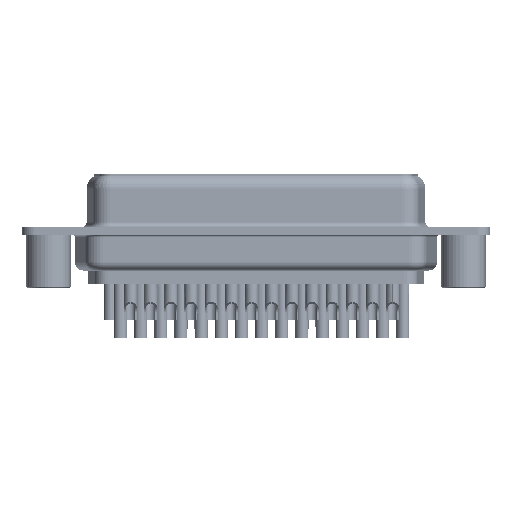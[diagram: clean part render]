
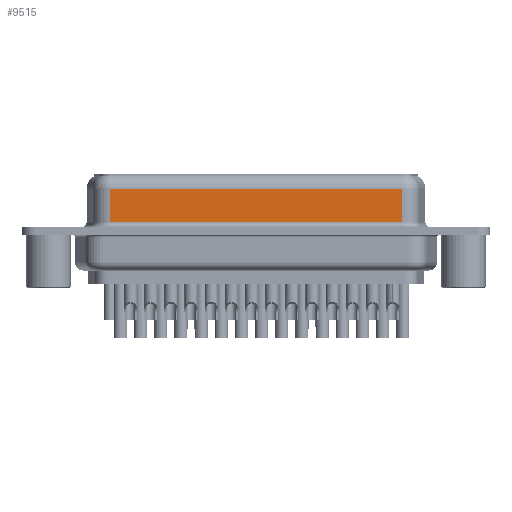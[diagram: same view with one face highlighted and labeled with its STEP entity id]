
A CAD part, front view. The second image highlights one B-rep face of the part: STEP entity #9515.
In plain terms, the highlighted planar face has unit normal (0, -1, 0).
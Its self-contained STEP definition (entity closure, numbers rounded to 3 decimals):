
#59 = CARTESIAN_POINT ( 'NONE',  ( 7.008, -3.95, 0.95 ) ) ;
#691 = DIRECTION ( 'NONE',  ( 0., 0., 1. ) ) ;
#1302 = EDGE_LOOP ( 'NONE', ( #9864, #17698, #5808, #7569 ) ) ;
#1887 = VECTOR ( 'NONE', #4143, 1000. ) ;
#4143 = DIRECTION ( 'NONE',  ( 0., 0., -1. ) ) ;
#5808 = ORIENTED_EDGE ( 'NONE', *, *, #12769, .T. ) ;
#6657 = EDGE_CURVE ( 'NONE', #9003, #11045, #10834, .T. ) ;
#7569 = ORIENTED_EDGE ( 'NONE', *, *, #13275, .T. ) ;
#9003 = VERTEX_POINT ( 'NONE', #17481 ) ;
#9515 = ADVANCED_FACE ( 'NONE', ( #14064 ), #31377, .F. ) ;
#9864 = ORIENTED_EDGE ( 'NONE', *, *, #21808, .F. ) ;
#10677 = VECTOR ( 'NONE', #25814, 1000. ) ;
#10834 = LINE ( 'NONE', #31301, #27037 ) ;
#11045 = VERTEX_POINT ( 'NONE', #33156 ) ;
#11209 = DIRECTION ( 'NONE',  ( -1., 0., 0. ) ) ;
#12769 = EDGE_CURVE ( 'NONE', #11045, #16908, #17257, .T. ) ;
#13275 = EDGE_CURVE ( 'NONE', #16908, #16281, #23882, .T. ) ;
#14064 = FACE_OUTER_BOUND ( 'NONE', #1302, .T. ) ;
#16281 = VERTEX_POINT ( 'NONE', #36037 ) ;
#16908 = VERTEX_POINT ( 'NONE', #59 ) ;
#17257 = LINE ( 'NONE', #30852, #10677 ) ;
#17427 = DIRECTION ( 'NONE',  ( 0., 1., 0. ) ) ;
#17481 = CARTESIAN_POINT ( 'NONE',  ( 40.032, -3.95, 4.7 ) ) ;
#17698 = ORIENTED_EDGE ( 'NONE', *, *, #6657, .T. ) ;
#18462 = LINE ( 'NONE', #24735, #1887 ) ;
#21808 = EDGE_CURVE ( 'NONE', #9003, #16281, #18462, .T. ) ;
#23150 = CARTESIAN_POINT ( 'NONE',  ( 40.032, -3.95, 0.95 ) ) ;
#23882 = LINE ( 'NONE', #23150, #28459 ) ;
#24735 = CARTESIAN_POINT ( 'NONE',  ( 40.032, -3.95, 6.45 ) ) ;
#25814 = DIRECTION ( 'NONE',  ( 0., 0., -1. ) ) ;
#26516 = AXIS2_PLACEMENT_3D ( 'NONE', #34544, #17427, #691 ) ;
#27037 = VECTOR ( 'NONE', #11209, 1000. ) ;
#28459 = VECTOR ( 'NONE', #32262, 1000. ) ;
#30852 = CARTESIAN_POINT ( 'NONE',  ( 7.008, -3.95, 6.45 ) ) ;
#31301 = CARTESIAN_POINT ( 'NONE',  ( 40.032, -3.95, 4.7 ) ) ;
#31377 = PLANE ( 'NONE',  #26516 ) ;
#32262 = DIRECTION ( 'NONE',  ( 1., 0., 0. ) ) ;
#33156 = CARTESIAN_POINT ( 'NONE',  ( 7.008, -3.95, 4.7 ) ) ;
#34544 = CARTESIAN_POINT ( 'NONE',  ( 40.032, -3.95, 6.45 ) ) ;
#36037 = CARTESIAN_POINT ( 'NONE',  ( 40.032, -3.95, 0.95 ) ) ;
